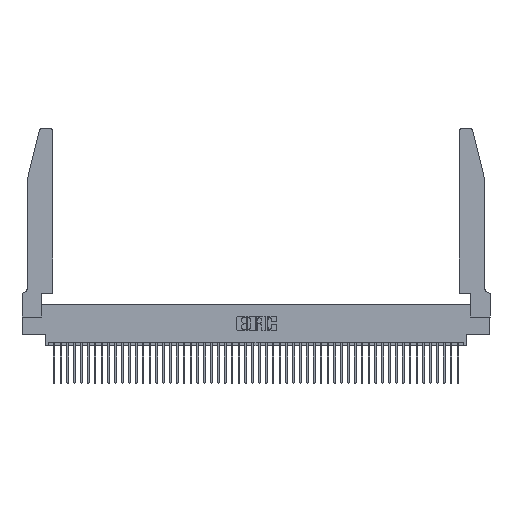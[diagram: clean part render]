
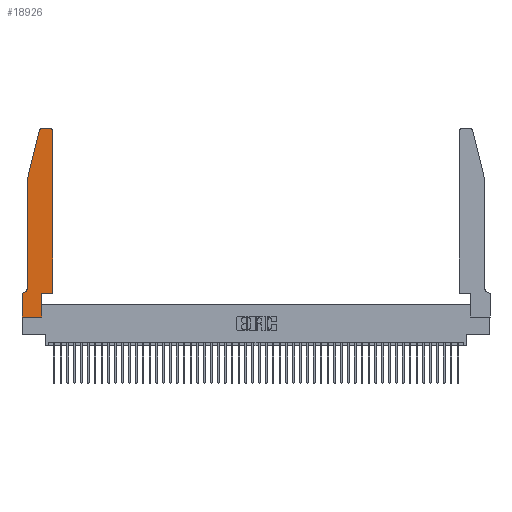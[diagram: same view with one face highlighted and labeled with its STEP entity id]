
A CAD part, top view. The second image highlights one B-rep face of the part: STEP entity #18926.
In plain terms, the highlighted planar face has unit normal (0, 0, 1).
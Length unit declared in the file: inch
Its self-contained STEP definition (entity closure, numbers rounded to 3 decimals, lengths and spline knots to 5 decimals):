
#96 = ORIENTED_EDGE ( 'NONE', *, *, #29601, .T. ) ;
#1104 = VERTEX_POINT ( 'NONE', #24933 ) ;
#1649 = EDGE_CURVE ( 'NONE', #36158, #19669, #20568, .T. ) ;
#2621 = DIRECTION ( 'NONE',  ( 1., 0., 0. ) ) ;
#3133 = ORIENTED_EDGE ( 'NONE', *, *, #47964, .T. ) ;
#3225 = VERTEX_POINT ( 'NONE', #18988 ) ;
#3372 = EDGE_CURVE ( 'NONE', #3978, #1104, #39318, .T. ) ;
#3582 = DIRECTION ( 'NONE',  ( 0., 0., -1. ) ) ;
#3588 = LINE ( 'NONE', #28007, #41924 ) ;
#3978 = VERTEX_POINT ( 'NONE', #38408 ) ;
#4039 = VERTEX_POINT ( 'NONE', #31266 ) ;
#4558 = EDGE_CURVE ( 'NONE', #26916, #4039, #6846, .T. ) ;
#5373 = CARTESIAN_POINT ( 'NONE',  ( 0.4205, 2.72, 0.37 ) ) ;
#6845 = ORIENTED_EDGE ( 'NONE', *, *, #1649, .T. ) ;
#6846 = LINE ( 'NONE', #18714, #18334 ) ;
#8802 = VECTOR ( 'NONE', #38623, 39.37008 ) ;
#9283 = DIRECTION ( 'NONE',  ( 1., 0., 0. ) ) ;
#9752 = VERTEX_POINT ( 'NONE', #31618 ) ;
#10369 = VECTOR ( 'NONE', #12549, 39.37008 ) ;
#10672 = DIRECTION ( 'NONE',  ( -0.239, -0.971, 0. ) ) ;
#12482 = CIRCLE ( 'NONE', #39973, 0.03 ) ;
#12517 = AXIS2_PLACEMENT_3D ( 'NONE', #17141, #20999, #47638 ) ;
#12549 = DIRECTION ( 'NONE',  ( 0., 1., 0. ) ) ;
#13314 = PLANE ( 'NONE',  #12517 ) ;
#14678 = VERTEX_POINT ( 'NONE', #21152 ) ;
#14820 = VERTEX_POINT ( 'NONE', #44754 ) ;
#15482 = LINE ( 'NONE', #31200, #43478 ) ;
#16009 = DIRECTION ( 'NONE',  ( 1., 0., 0. ) ) ;
#16593 = CARTESIAN_POINT ( 'NONE',  ( 0., 0., 0.37 ) ) ;
#17141 = CARTESIAN_POINT ( 'NONE',  ( 0., 0.35, 0.37 ) ) ;
#18334 = VECTOR ( 'NONE', #45344, 39.37008 ) ;
#18714 = CARTESIAN_POINT ( 'NONE',  ( 0.0755, 2., 0.37 ) ) ;
#18729 = VERTEX_POINT ( 'NONE', #27333 ) ;
#18926 = ADVANCED_FACE ( 'NONE', ( #22541 ), #13314, .T. ) ;
#18988 = CARTESIAN_POINT ( 'NONE',  ( 0.0055, 0.35, 0.37 ) ) ;
#19641 = CARTESIAN_POINT ( 'NONE',  ( 0., 0., 0.37 ) ) ;
#19669 = VERTEX_POINT ( 'NONE', #37434 ) ;
#20067 = CARTESIAN_POINT ( 'NONE',  ( 0.4505, 0.35, 0.37 ) ) ;
#20264 = EDGE_LOOP ( 'NONE', ( #3133, #96, #49284, #31508, #36124, #48065, #21729, #42776, #41952, #35355, #6845, #38046 ) ) ;
#20352 = VECTOR ( 'NONE', #38824, 39.37008 ) ;
#20568 = LINE ( 'NONE', #20067, #10369 ) ;
#20999 = DIRECTION ( 'NONE',  ( 0., 0., 1. ) ) ;
#21152 = CARTESIAN_POINT ( 'NONE',  ( 0.2865, 0.35, 0.37 ) ) ;
#21729 = ORIENTED_EDGE ( 'NONE', *, *, #36231, .T. ) ;
#22541 = FACE_OUTER_BOUND ( 'NONE', #20264, .T. ) ;
#23553 = EDGE_CURVE ( 'NONE', #3225, #35734, #3588, .T. ) ;
#24104 = DIRECTION ( 'NONE',  ( 0., -1., 0. ) ) ;
#24169 = CARTESIAN_POINT ( 'NONE',  ( 0.2605, 2.75, 0.37 ) ) ;
#24933 = CARTESIAN_POINT ( 'NONE',  ( 0.2865, 0., 0.37 ) ) ;
#25235 = EDGE_CURVE ( 'NONE', #18729, #26916, #38765, .T. ) ;
#25602 = AXIS2_PLACEMENT_3D ( 'NONE', #48434, #25634, #2621 ) ;
#25634 = DIRECTION ( 'NONE',  ( 0., 0., 1. ) ) ;
#26579 = CARTESIAN_POINT ( 'NONE',  ( 0.0055, 0.42, 0.37 ) ) ;
#26916 = VERTEX_POINT ( 'NONE', #48415 ) ;
#27333 = CARTESIAN_POINT ( 'NONE',  ( 0.25487, 2.72718, 0.37 ) ) ;
#27614 = CARTESIAN_POINT ( 'NONE',  ( 0.4505, 0.35, 0.37 ) ) ;
#28007 = CARTESIAN_POINT ( 'NONE',  ( 0.0755, 0.35, 0.37 ) ) ;
#28583 = VECTOR ( 'NONE', #31857, 39.37008 ) ;
#28645 = VECTOR ( 'NONE', #10672, 39.37008 ) ;
#29601 = EDGE_CURVE ( 'NONE', #14820, #18729, #42468, .T. ) ;
#29784 = LINE ( 'NONE', #24169, #28583 ) ;
#30437 = DIRECTION ( 'NONE',  ( -1., 0., 0. ) ) ;
#30484 = LINE ( 'NONE', #42325, #20352 ) ;
#31200 = CARTESIAN_POINT ( 'NONE',  ( 0.4505, 0.35, 0.37 ) ) ;
#31266 = CARTESIAN_POINT ( 'NONE',  ( 0.0755, 0.42, 0.37 ) ) ;
#31508 = ORIENTED_EDGE ( 'NONE', *, *, #4558, .T. ) ;
#31618 = CARTESIAN_POINT ( 'NONE',  ( 0.4205, 2.75, 0.37 ) ) ;
#31857 = DIRECTION ( 'NONE',  ( -1., 0., 0. ) ) ;
#32214 = DIRECTION ( 'NONE',  ( 0., 0., 1. ) ) ;
#32832 = CARTESIAN_POINT ( 'NONE',  ( 0., 0.35, 0.37 ) ) ;
#35355 = ORIENTED_EDGE ( 'NONE', *, *, #47862, .T. ) ;
#35734 = VERTEX_POINT ( 'NONE', #32832 ) ;
#36124 = ORIENTED_EDGE ( 'NONE', *, *, #48842, .T. ) ;
#36158 = VERTEX_POINT ( 'NONE', #27614 ) ;
#36231 = EDGE_CURVE ( 'NONE', #35734, #3978, #42707, .T. ) ;
#37039 = CARTESIAN_POINT ( 'NONE',  ( 0.0755, 2., 0.37 ) ) ;
#37434 = CARTESIAN_POINT ( 'NONE',  ( 0.4505, 2.72, 0.37 ) ) ;
#38046 = ORIENTED_EDGE ( 'NONE', *, *, #47035, .T. ) ;
#38408 = CARTESIAN_POINT ( 'NONE',  ( 0., 0., 0.37 ) ) ;
#38623 = DIRECTION ( 'NONE',  ( 1., 0., 0. ) ) ;
#38765 = LINE ( 'NONE', #37039, #28645 ) ;
#38824 = DIRECTION ( 'NONE',  ( 0., 1., 0. ) ) ;
#39226 = EDGE_CURVE ( 'NONE', #1104, #14678, #30484, .T. ) ;
#39318 = LINE ( 'NONE', #19641, #8802 ) ;
#39795 = CIRCLE ( 'NONE', #45420, 0.07 ) ;
#39973 = AXIS2_PLACEMENT_3D ( 'NONE', #5373, #32214, #9283 ) ;
#41539 = VECTOR ( 'NONE', #24104, 39.37008 ) ;
#41924 = VECTOR ( 'NONE', #46989, 39.37008 ) ;
#41952 = ORIENTED_EDGE ( 'NONE', *, *, #39226, .T. ) ;
#42325 = CARTESIAN_POINT ( 'NONE',  ( 0.2865, 0.35, 0.37 ) ) ;
#42468 = CIRCLE ( 'NONE', #25602, 0.03 ) ;
#42707 = LINE ( 'NONE', #16593, #41539 ) ;
#42776 = ORIENTED_EDGE ( 'NONE', *, *, #3372, .T. ) ;
#43478 = VECTOR ( 'NONE', #16009, 39.37008 ) ;
#44754 = CARTESIAN_POINT ( 'NONE',  ( 0.284, 2.75, 0.37 ) ) ;
#45344 = DIRECTION ( 'NONE',  ( 0., -1., 0. ) ) ;
#45420 = AXIS2_PLACEMENT_3D ( 'NONE', #26579, #3582, #30437 ) ;
#46989 = DIRECTION ( 'NONE',  ( -1., 0., 0. ) ) ;
#47035 = EDGE_CURVE ( 'NONE', #19669, #9752, #12482, .T. ) ;
#47638 = DIRECTION ( 'NONE',  ( 1., 0., 0. ) ) ;
#47862 = EDGE_CURVE ( 'NONE', #14678, #36158, #15482, .T. ) ;
#47964 = EDGE_CURVE ( 'NONE', #9752, #14820, #29784, .T. ) ;
#48065 = ORIENTED_EDGE ( 'NONE', *, *, #23553, .T. ) ;
#48415 = CARTESIAN_POINT ( 'NONE',  ( 0.0755, 2., 0.37 ) ) ;
#48434 = CARTESIAN_POINT ( 'NONE',  ( 0.284, 2.72, 0.37 ) ) ;
#48842 = EDGE_CURVE ( 'NONE', #4039, #3225, #39795, .T. ) ;
#49284 = ORIENTED_EDGE ( 'NONE', *, *, #25235, .T. ) ;
